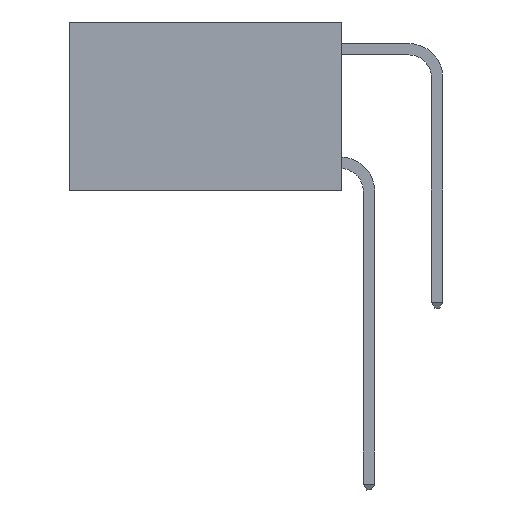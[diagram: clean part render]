
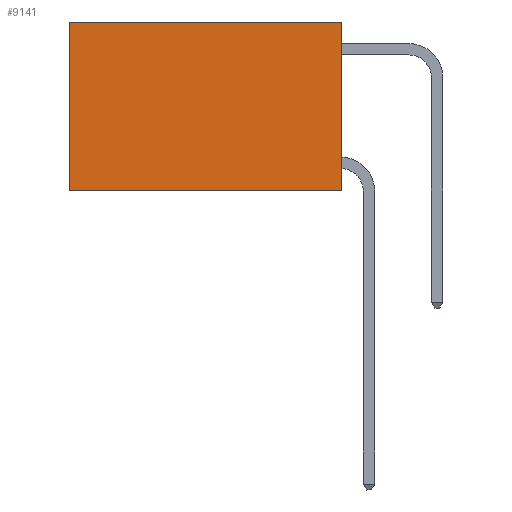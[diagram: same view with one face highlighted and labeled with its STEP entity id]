
A CAD part, left-side view. The second image highlights one B-rep face of the part: STEP entity #9141.
In plain terms, the highlighted planar face has unit normal (-1, 0, 0).
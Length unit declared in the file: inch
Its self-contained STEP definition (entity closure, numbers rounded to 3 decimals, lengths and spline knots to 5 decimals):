
#538 = CARTESIAN_POINT ( 'NONE',  ( 0.2625, 0., 0. ) ) ;
#882 = CARTESIAN_POINT ( 'NONE',  ( 0.2625, 0., -0.37 ) ) ;
#910 = DIRECTION ( 'NONE',  ( 1., 0., 0. ) ) ;
#1031 = FACE_OUTER_BOUND ( 'NONE', #3682, .T. ) ;
#1398 = CARTESIAN_POINT ( 'NONE',  ( 0.2625, 0.6, 0. ) ) ;
#1953 = VERTEX_POINT ( 'NONE', #1398 ) ;
#1996 = CARTESIAN_POINT ( 'NONE',  ( 0.2625, 0., 0. ) ) ;
#2160 = LINE ( 'NONE', #538, #6574 ) ;
#2329 = LINE ( 'NONE', #4916, #8400 ) ;
#3096 = DIRECTION ( 'NONE',  ( 0., 0., -1. ) ) ;
#3682 = EDGE_LOOP ( 'NONE', ( #4900, #9014, #6340, #10427 ) ) ;
#4330 = EDGE_CURVE ( 'NONE', #5657, #8337, #4811, .T. ) ;
#4453 = VECTOR ( 'NONE', #5651, 39.37008 ) ;
#4567 = VERTEX_POINT ( 'NONE', #8914 ) ;
#4764 = EDGE_CURVE ( 'NONE', #1953, #4567, #2329, .T. ) ;
#4811 = LINE ( 'NONE', #8218, #8472 ) ;
#4819 = EDGE_CURVE ( 'NONE', #5657, #1953, #2160, .T. ) ;
#4900 = ORIENTED_EDGE ( 'NONE', *, *, #4764, .T. ) ;
#4916 = CARTESIAN_POINT ( 'NONE',  ( 0.2625, 0.6, 0. ) ) ;
#5651 = DIRECTION ( 'NONE',  ( 0., 1., 0. ) ) ;
#5657 = VERTEX_POINT ( 'NONE', #1996 ) ;
#6167 = EDGE_CURVE ( 'NONE', #8337, #4567, #10064, .T. ) ;
#6340 = ORIENTED_EDGE ( 'NONE', *, *, #4330, .F. ) ;
#6496 = DIRECTION ( 'NONE',  ( 0., 0., -1. ) ) ;
#6574 = VECTOR ( 'NONE', #10994, 39.37008 ) ;
#8218 = CARTESIAN_POINT ( 'NONE',  ( 0.2625, 0., 0. ) ) ;
#8337 = VERTEX_POINT ( 'NONE', #882 ) ;
#8400 = VECTOR ( 'NONE', #6496, 39.37008 ) ;
#8472 = VECTOR ( 'NONE', #3096, 39.37008 ) ;
#8668 = CARTESIAN_POINT ( 'NONE',  ( 0.2625, 0., 0. ) ) ;
#8828 = PLANE ( 'NONE',  #10544 ) ;
#8914 = CARTESIAN_POINT ( 'NONE',  ( 0.2625, 0.6, -0.37 ) ) ;
#9014 = ORIENTED_EDGE ( 'NONE', *, *, #6167, .F. ) ;
#9141 = ADVANCED_FACE ( 'NONE', ( #1031 ), #8828, .F. ) ;
#10064 = LINE ( 'NONE', #10942, #4453 ) ;
#10427 = ORIENTED_EDGE ( 'NONE', *, *, #4819, .T. ) ;
#10509 = DIRECTION ( 'NONE',  ( 0., 0., -1. ) ) ;
#10544 = AXIS2_PLACEMENT_3D ( 'NONE', #8668, #910, #10509 ) ;
#10942 = CARTESIAN_POINT ( 'NONE',  ( 0.2625, 0., -0.37 ) ) ;
#10994 = DIRECTION ( 'NONE',  ( 0., 1., 0. ) ) ;
